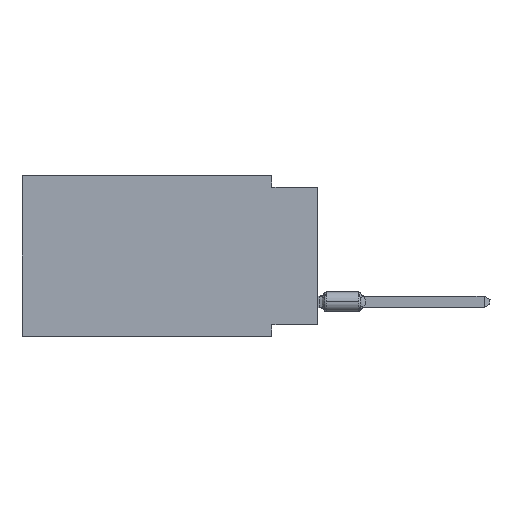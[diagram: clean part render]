
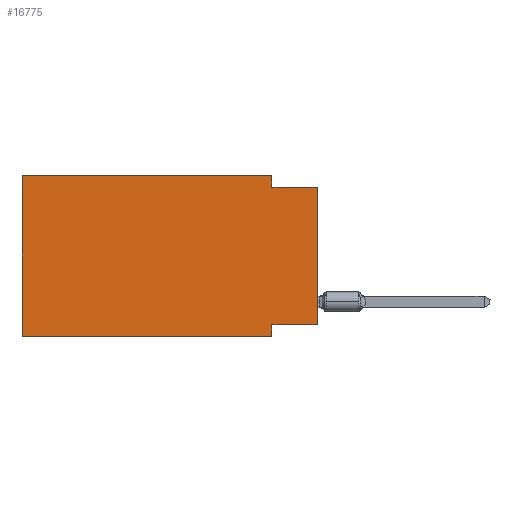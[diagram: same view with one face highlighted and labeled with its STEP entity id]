
A CAD part, left-side view. The second image highlights one B-rep face of the part: STEP entity #16775.
In plain terms, the highlighted planar face has unit normal (-1, 0, 0).
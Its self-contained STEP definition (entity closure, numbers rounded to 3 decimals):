
#1174 = VERTEX_POINT ( 'NONE', #16660 ) ;
#1359 = PLANE ( 'NONE',  #29301 ) ;
#1526 = DIRECTION ( 'NONE',  ( 0., -1., 0. ) ) ;
#1721 = CARTESIAN_POINT ( 'NONE',  ( 0., 0., 0. ) ) ;
#2062 = VECTOR ( 'NONE', #20209, 1000. ) ;
#2090 = VECTOR ( 'NONE', #1526, 1000. ) ;
#2701 = EDGE_CURVE ( 'NONE', #24599, #22042, #22754, .T. ) ;
#3318 = CARTESIAN_POINT ( 'NONE',  ( 0., 2.54, -8.255 ) ) ;
#3358 = ORIENTED_EDGE ( 'NONE', *, *, #33414, .F. ) ;
#3771 = VECTOR ( 'NONE', #40063, 1000. ) ;
#4779 = FACE_OUTER_BOUND ( 'NONE', #41922, .T. ) ;
#6480 = VECTOR ( 'NONE', #31659, 1000. ) ;
#7059 = ORIENTED_EDGE ( 'NONE', *, *, #2701, .F. ) ;
#7590 = VECTOR ( 'NONE', #40504, 1000. ) ;
#7980 = DIRECTION ( 'NONE',  ( 0., 0., -1. ) ) ;
#9913 = CARTESIAN_POINT ( 'NONE',  ( 0., 0., -8.255 ) ) ;
#10377 = CARTESIAN_POINT ( 'NONE',  ( 0., 2.54, 0. ) ) ;
#10978 = CARTESIAN_POINT ( 'NONE',  ( 0., 16.383, 0. ) ) ;
#13656 = CARTESIAN_POINT ( 'NONE',  ( 0., 16.383, 0. ) ) ;
#13821 = VERTEX_POINT ( 'NONE', #3318 ) ;
#15157 = CARTESIAN_POINT ( 'NONE',  ( 0., 0., -0.635 ) ) ;
#15795 = CARTESIAN_POINT ( 'NONE',  ( 0., 0., -8.255 ) ) ;
#15909 = DIRECTION ( 'NONE',  ( 0., 0., 1. ) ) ;
#16660 = CARTESIAN_POINT ( 'NONE',  ( 0., 2.54, -0.635 ) ) ;
#16775 = ADVANCED_FACE ( 'NONE', ( #4779 ), #1359, .F. ) ;
#18481 = ORIENTED_EDGE ( 'NONE', *, *, #25027, .F. ) ;
#20209 = DIRECTION ( 'NONE',  ( 0., 1., 0. ) ) ;
#22042 = VERTEX_POINT ( 'NONE', #13656 ) ;
#22069 = LINE ( 'NONE', #22284, #2090 ) ;
#22173 = EDGE_CURVE ( 'NONE', #1174, #22534, #32326, .T. ) ;
#22284 = CARTESIAN_POINT ( 'NONE',  ( 0., 16.383, -8.89 ) ) ;
#22534 = VERTEX_POINT ( 'NONE', #15157 ) ;
#22754 = LINE ( 'NONE', #43072, #31369 ) ;
#22933 = LINE ( 'NONE', #1721, #24344 ) ;
#23235 = CARTESIAN_POINT ( 'NONE',  ( 0., 2.54, 0. ) ) ;
#23615 = ORIENTED_EDGE ( 'NONE', *, *, #26005, .F. ) ;
#24344 = VECTOR ( 'NONE', #43461, 1000. ) ;
#24599 = VERTEX_POINT ( 'NONE', #43310 ) ;
#24799 = CARTESIAN_POINT ( 'NONE',  ( 0., 2.54, -8.89 ) ) ;
#24991 = EDGE_CURVE ( 'NONE', #27489, #22534, #22933, .T. ) ;
#25024 = LINE ( 'NONE', #24799, #6480 ) ;
#25027 = EDGE_CURVE ( 'NONE', #22042, #38680, #30453, .T. ) ;
#26005 = EDGE_CURVE ( 'NONE', #13821, #41085, #25024, .T. ) ;
#26120 = CARTESIAN_POINT ( 'NONE',  ( 0., 0., -0.635 ) ) ;
#27271 = CARTESIAN_POINT ( 'NONE',  ( 0., 16.383, 0. ) ) ;
#27489 = VERTEX_POINT ( 'NONE', #15795 ) ;
#28332 = EDGE_CURVE ( 'NONE', #38680, #1174, #38653, .T. ) ;
#28360 = VECTOR ( 'NONE', #31128, 1000. ) ;
#29301 = AXIS2_PLACEMENT_3D ( 'NONE', #10978, #31946, #7980 ) ;
#30137 = ORIENTED_EDGE ( 'NONE', *, *, #22173, .F. ) ;
#30453 = LINE ( 'NONE', #27271, #7590 ) ;
#30476 = ORIENTED_EDGE ( 'NONE', *, *, #28332, .F. ) ;
#30701 = LINE ( 'NONE', #9913, #2062 ) ;
#31128 = DIRECTION ( 'NONE',  ( 0., 0., -1. ) ) ;
#31369 = VECTOR ( 'NONE', #15909, 1000. ) ;
#31659 = DIRECTION ( 'NONE',  ( 0., 0., -1. ) ) ;
#31946 = DIRECTION ( 'NONE',  ( 1., 0., 0. ) ) ;
#32326 = LINE ( 'NONE', #26120, #3771 ) ;
#33337 = CARTESIAN_POINT ( 'NONE',  ( 0., 2.54, -8.89 ) ) ;
#33414 = EDGE_CURVE ( 'NONE', #27489, #13821, #30701, .T. ) ;
#35724 = EDGE_CURVE ( 'NONE', #24599, #41085, #22069, .T. ) ;
#38653 = LINE ( 'NONE', #10377, #28360 ) ;
#38680 = VERTEX_POINT ( 'NONE', #23235 ) ;
#39949 = ORIENTED_EDGE ( 'NONE', *, *, #35724, .T. ) ;
#40063 = DIRECTION ( 'NONE',  ( 0., -1., 0. ) ) ;
#40504 = DIRECTION ( 'NONE',  ( 0., -1., 0. ) ) ;
#40512 = ORIENTED_EDGE ( 'NONE', *, *, #24991, .T. ) ;
#41085 = VERTEX_POINT ( 'NONE', #33337 ) ;
#41922 = EDGE_LOOP ( 'NONE', ( #40512, #30137, #30476, #18481, #7059, #39949, #23615, #3358 ) ) ;
#43072 = CARTESIAN_POINT ( 'NONE',  ( 0., 16.383, 0. ) ) ;
#43310 = CARTESIAN_POINT ( 'NONE',  ( 0., 16.383, -8.89 ) ) ;
#43461 = DIRECTION ( 'NONE',  ( 0., 0., 1. ) ) ;
